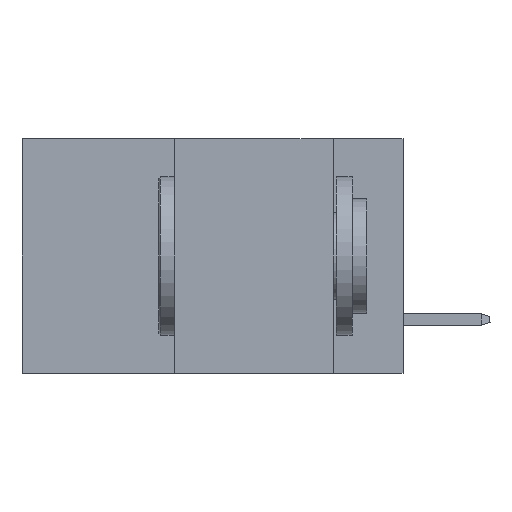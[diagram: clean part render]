
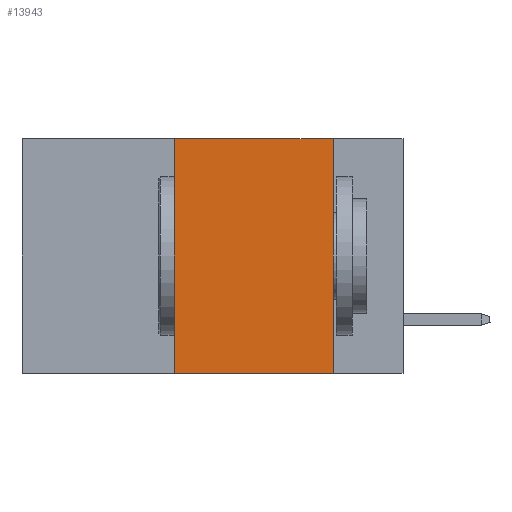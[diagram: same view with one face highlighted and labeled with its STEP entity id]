
A CAD part, left-side view. The second image highlights one B-rep face of the part: STEP entity #13943.
In plain terms, the highlighted planar face has unit normal (-1, 0, 0).
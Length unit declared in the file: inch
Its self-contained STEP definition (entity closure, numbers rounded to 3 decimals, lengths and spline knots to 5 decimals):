
#88 = VECTOR ( 'NONE', #10233, 39.37008 ) ;
#2275 = LINE ( 'NONE', #31478, #88 ) ;
#4649 = LINE ( 'NONE', #29210, #27684 ) ;
#5290 = DIRECTION ( 'NONE',  ( 0., -1., 0. ) ) ;
#5669 = AXIS2_PLACEMENT_3D ( 'NONE', #28254, #20109, #25782 ) ;
#6456 = ORIENTED_EDGE ( 'NONE', *, *, #13247, .F. ) ;
#7096 = CARTESIAN_POINT ( 'NONE',  ( 0., 0.11, -0.37 ) ) ;
#7788 = LINE ( 'NONE', #15893, #23711 ) ;
#8427 = VECTOR ( 'NONE', #5290, 39.37008 ) ;
#10233 = DIRECTION ( 'NONE',  ( 0., 0., -1. ) ) ;
#12801 = ORIENTED_EDGE ( 'NONE', *, *, #14988, .F. ) ;
#13247 = EDGE_CURVE ( 'NONE', #29405, #29330, #4649, .T. ) ;
#13720 = EDGE_CURVE ( 'NONE', #27536, #32884, #26677, .T. ) ;
#13943 = ADVANCED_FACE ( 'NONE', ( #33568 ), #28076, .F. ) ;
#14988 = EDGE_CURVE ( 'NONE', #27536, #29405, #7788, .T. ) ;
#15893 = CARTESIAN_POINT ( 'NONE',  ( 0., 0.36, 0. ) ) ;
#16104 = DIRECTION ( 'NONE',  ( 0., -1., 0. ) ) ;
#16963 = EDGE_CURVE ( 'NONE', #29330, #32884, #2275, .T. ) ;
#18547 = EDGE_LOOP ( 'NONE', ( #22083, #6456, #12801, #29004 ) ) ;
#19801 = CARTESIAN_POINT ( 'NONE',  ( 0., 0.11, 0. ) ) ;
#20109 = DIRECTION ( 'NONE',  ( 1., 0., 0. ) ) ;
#22083 = ORIENTED_EDGE ( 'NONE', *, *, #16963, .F. ) ;
#23518 = CARTESIAN_POINT ( 'NONE',  ( 0., 0.36, 0. ) ) ;
#23711 = VECTOR ( 'NONE', #24193, 39.37008 ) ;
#24193 = DIRECTION ( 'NONE',  ( 0., 0., 1. ) ) ;
#25782 = DIRECTION ( 'NONE',  ( 0., 0., -1. ) ) ;
#26621 = CARTESIAN_POINT ( 'NONE',  ( 0., 0.36, -0.37 ) ) ;
#26677 = LINE ( 'NONE', #29501, #8427 ) ;
#27536 = VERTEX_POINT ( 'NONE', #26621 ) ;
#27684 = VECTOR ( 'NONE', #16104, 39.37008 ) ;
#28076 = PLANE ( 'NONE',  #5669 ) ;
#28254 = CARTESIAN_POINT ( 'NONE',  ( 0., 0.6, 0. ) ) ;
#29004 = ORIENTED_EDGE ( 'NONE', *, *, #13720, .T. ) ;
#29210 = CARTESIAN_POINT ( 'NONE',  ( 0., 0.6, 0. ) ) ;
#29330 = VERTEX_POINT ( 'NONE', #19801 ) ;
#29405 = VERTEX_POINT ( 'NONE', #23518 ) ;
#29501 = CARTESIAN_POINT ( 'NONE',  ( 0., 0.6, -0.37 ) ) ;
#31478 = CARTESIAN_POINT ( 'NONE',  ( 0., 0.11, 0. ) ) ;
#32884 = VERTEX_POINT ( 'NONE', #7096 ) ;
#33568 = FACE_OUTER_BOUND ( 'NONE', #18547, .T. ) ;
